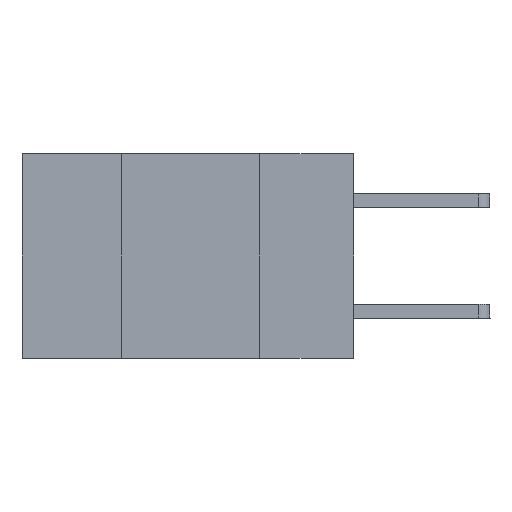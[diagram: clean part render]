
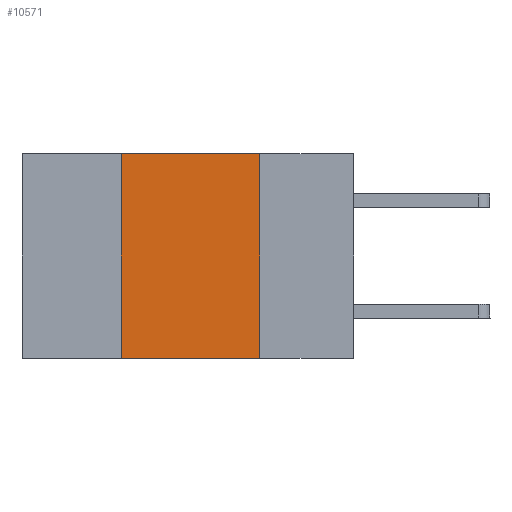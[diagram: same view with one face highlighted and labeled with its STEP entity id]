
A CAD part, left-side view. The second image highlights one B-rep face of the part: STEP entity #10571.
In plain terms, the highlighted planar face has unit normal (-1, 0, 0).
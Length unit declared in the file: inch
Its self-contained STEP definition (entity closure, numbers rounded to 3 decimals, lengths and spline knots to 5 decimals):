
#112 = CARTESIAN_POINT ( 'NONE',  ( 0., 0.6, 0. ) ) ;
#428 = LINE ( 'NONE', #7313, #3914 ) ;
#1150 = FACE_OUTER_BOUND ( 'NONE', #6770, .T. ) ;
#1635 = CARTESIAN_POINT ( 'NONE',  ( 0., 0.17, 0. ) ) ;
#1638 = ORIENTED_EDGE ( 'NONE', *, *, #13289, .F. ) ;
#2203 = LINE ( 'NONE', #6394, #12124 ) ;
#2412 = EDGE_CURVE ( 'NONE', #10690, #4671, #4286, .T. ) ;
#3185 = VECTOR ( 'NONE', #3653, 39.37008 ) ;
#3360 = ORIENTED_EDGE ( 'NONE', *, *, #4322, .T. ) ;
#3430 = CARTESIAN_POINT ( 'NONE',  ( 0., 0.42, 0. ) ) ;
#3653 = DIRECTION ( 'NONE',  ( 0., -1., 0. ) ) ;
#3788 = ORIENTED_EDGE ( 'NONE', *, *, #4754, .F. ) ;
#3914 = VECTOR ( 'NONE', #4630, 39.37008 ) ;
#4286 = LINE ( 'NONE', #8457, #10349 ) ;
#4292 = CARTESIAN_POINT ( 'NONE',  ( 0., 0.17, -0.37 ) ) ;
#4315 = DIRECTION ( 'NONE',  ( 1., 0., 0. ) ) ;
#4322 = EDGE_CURVE ( 'NONE', #10690, #7765, #12999, .T. ) ;
#4569 = AXIS2_PLACEMENT_3D ( 'NONE', #112, #4315, #8485 ) ;
#4572 = CARTESIAN_POINT ( 'NONE',  ( 0., 0.42, -0.37 ) ) ;
#4630 = DIRECTION ( 'NONE',  ( 0., -1., 0. ) ) ;
#4671 = VERTEX_POINT ( 'NONE', #3430 ) ;
#4746 = CARTESIAN_POINT ( 'NONE',  ( 0., 0.6, -0.37 ) ) ;
#4754 = EDGE_CURVE ( 'NONE', #8940, #7765, #2203, .T. ) ;
#5358 = PLANE ( 'NONE',  #4569 ) ;
#6394 = CARTESIAN_POINT ( 'NONE',  ( 0., 0.17, 0. ) ) ;
#6770 = EDGE_LOOP ( 'NONE', ( #3788, #1638, #9053, #3360 ) ) ;
#7313 = CARTESIAN_POINT ( 'NONE',  ( 0., 0.6, 0. ) ) ;
#7765 = VERTEX_POINT ( 'NONE', #4292 ) ;
#8457 = CARTESIAN_POINT ( 'NONE',  ( 0., 0.42, 0. ) ) ;
#8485 = DIRECTION ( 'NONE',  ( 0., 0., -1. ) ) ;
#8940 = VERTEX_POINT ( 'NONE', #1635 ) ;
#9053 = ORIENTED_EDGE ( 'NONE', *, *, #2412, .F. ) ;
#10349 = VECTOR ( 'NONE', #11599, 39.37008 ) ;
#10541 = DIRECTION ( 'NONE',  ( 0., 0., -1. ) ) ;
#10571 = ADVANCED_FACE ( 'NONE', ( #1150 ), #5358, .F. ) ;
#10690 = VERTEX_POINT ( 'NONE', #4572 ) ;
#11599 = DIRECTION ( 'NONE',  ( 0., 0., 1. ) ) ;
#12124 = VECTOR ( 'NONE', #10541, 39.37008 ) ;
#12999 = LINE ( 'NONE', #4746, #3185 ) ;
#13289 = EDGE_CURVE ( 'NONE', #4671, #8940, #428, .T. ) ;
